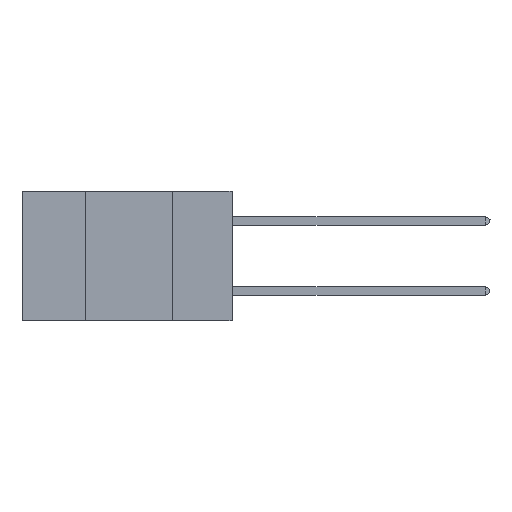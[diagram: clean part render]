
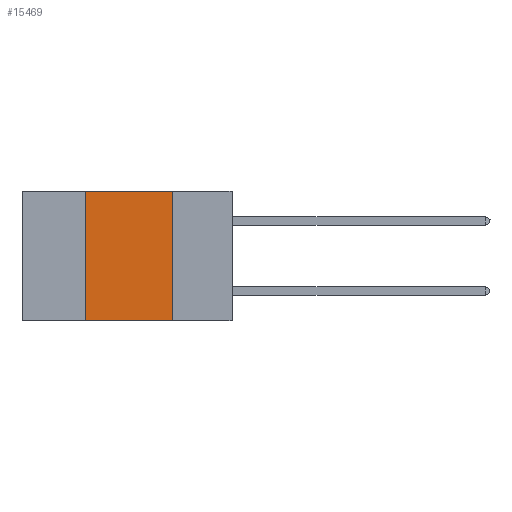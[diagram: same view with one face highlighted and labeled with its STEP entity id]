
A CAD part, left-side view. The second image highlights one B-rep face of the part: STEP entity #15469.
In plain terms, the highlighted planar face has unit normal (-1, 0, 0).
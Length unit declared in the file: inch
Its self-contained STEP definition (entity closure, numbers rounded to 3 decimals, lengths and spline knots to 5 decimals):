
#64 = CARTESIAN_POINT ( 'NONE',  ( 0., 0.17, -0.37 ) ) ;
#935 = CARTESIAN_POINT ( 'NONE',  ( 0., 0.6, 0. ) ) ;
#940 = VECTOR ( 'NONE', #13715, 39.37008 ) ;
#1057 = VECTOR ( 'NONE', #3072, 39.37008 ) ;
#1217 = LINE ( 'NONE', #7935, #940 ) ;
#1375 = ORIENTED_EDGE ( 'NONE', *, *, #8973, .F. ) ;
#2244 = VECTOR ( 'NONE', #11609, 39.37008 ) ;
#2280 = CARTESIAN_POINT ( 'NONE',  ( 0., 0.6, 0. ) ) ;
#3028 = ORIENTED_EDGE ( 'NONE', *, *, #3649, .T. ) ;
#3069 = EDGE_CURVE ( 'NONE', #12353, #17108, #1217, .T. ) ;
#3072 = DIRECTION ( 'NONE',  ( 0., -1., 0. ) ) ;
#3649 = EDGE_CURVE ( 'NONE', #12353, #17243, #11586, .T. ) ;
#3730 = DIRECTION ( 'NONE',  ( 1., 0., 0. ) ) ;
#4925 = DIRECTION ( 'NONE',  ( 0., -1., 0. ) ) ;
#5068 = LINE ( 'NONE', #14426, #2244 ) ;
#5204 = EDGE_CURVE ( 'NONE', #6620, #17243, #5068, .T. ) ;
#6620 = VERTEX_POINT ( 'NONE', #11409 ) ;
#7898 = PLANE ( 'NONE',  #10627 ) ;
#7935 = CARTESIAN_POINT ( 'NONE',  ( 0., 0.42, 0. ) ) ;
#8087 = FACE_OUTER_BOUND ( 'NONE', #9132, .T. ) ;
#8973 = EDGE_CURVE ( 'NONE', #17108, #6620, #13264, .T. ) ;
#9132 = EDGE_LOOP ( 'NONE', ( #12992, #1375, #15834, #3028 ) ) ;
#10139 = CARTESIAN_POINT ( 'NONE',  ( 0., 0.6, -0.37 ) ) ;
#10627 = AXIS2_PLACEMENT_3D ( 'NONE', #2280, #3730, #17427 ) ;
#11082 = VECTOR ( 'NONE', #4925, 39.37008 ) ;
#11409 = CARTESIAN_POINT ( 'NONE',  ( 0., 0.17, 0. ) ) ;
#11586 = LINE ( 'NONE', #10139, #1057 ) ;
#11609 = DIRECTION ( 'NONE',  ( 0., 0., -1. ) ) ;
#12353 = VERTEX_POINT ( 'NONE', #14906 ) ;
#12992 = ORIENTED_EDGE ( 'NONE', *, *, #5204, .F. ) ;
#13264 = LINE ( 'NONE', #935, #11082 ) ;
#13715 = DIRECTION ( 'NONE',  ( 0., 0., 1. ) ) ;
#14426 = CARTESIAN_POINT ( 'NONE',  ( 0., 0.17, 0. ) ) ;
#14906 = CARTESIAN_POINT ( 'NONE',  ( 0., 0.42, -0.37 ) ) ;
#15469 = ADVANCED_FACE ( 'NONE', ( #8087 ), #7898, .F. ) ;
#15834 = ORIENTED_EDGE ( 'NONE', *, *, #3069, .F. ) ;
#16327 = CARTESIAN_POINT ( 'NONE',  ( 0., 0.42, 0. ) ) ;
#17108 = VERTEX_POINT ( 'NONE', #16327 ) ;
#17243 = VERTEX_POINT ( 'NONE', #64 ) ;
#17427 = DIRECTION ( 'NONE',  ( 0., 0., -1. ) ) ;
